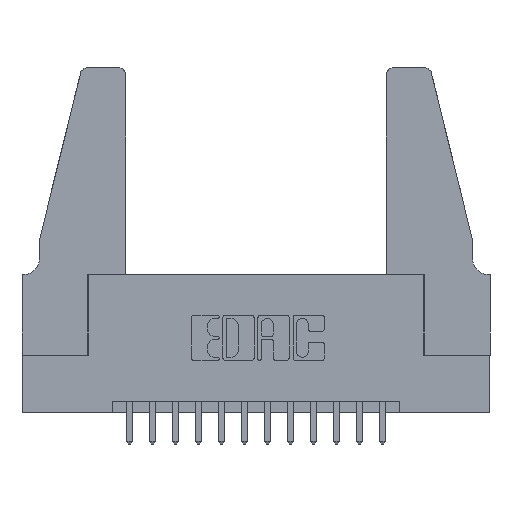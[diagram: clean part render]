
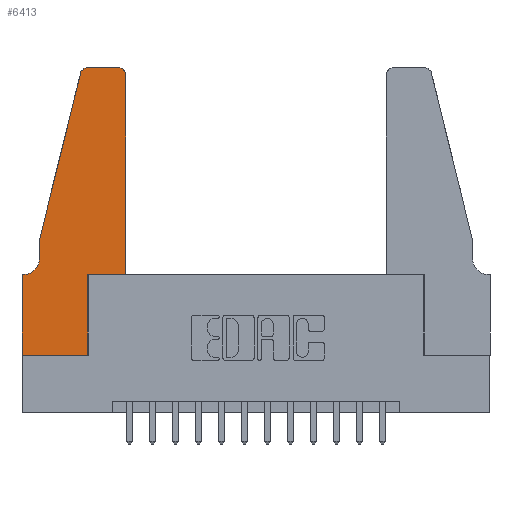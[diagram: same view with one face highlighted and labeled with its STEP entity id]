
A CAD part, top view. The second image highlights one B-rep face of the part: STEP entity #6413.
In plain terms, the highlighted planar face has unit normal (0, 0, 1).
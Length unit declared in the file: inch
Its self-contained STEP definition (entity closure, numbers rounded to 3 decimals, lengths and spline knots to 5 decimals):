
#133 = LINE ( 'NONE', #10324, #511 ) ;
#158 = EDGE_CURVE ( 'NONE', #15649, #6260, #133, .T. ) ;
#332 = EDGE_CURVE ( 'NONE', #9106, #620, #11481, .T. ) ;
#511 = VECTOR ( 'NONE', #10275, 39.37008 ) ;
#520 = VERTEX_POINT ( 'NONE', #4742 ) ;
#620 = VERTEX_POINT ( 'NONE', #6153 ) ;
#818 = EDGE_CURVE ( 'NONE', #14426, #7347, #7082, .T. ) ;
#876 = VECTOR ( 'NONE', #5156, 39.37008 ) ;
#976 = CARTESIAN_POINT ( 'NONE',  ( 0., 0.35, 0.37 ) ) ;
#988 = CARTESIAN_POINT ( 'NONE',  ( 0.4505, 0.35, 0.37 ) ) ;
#1846 = DIRECTION ( 'NONE',  ( 1., 0., 0. ) ) ;
#1961 = VECTOR ( 'NONE', #1846, 39.37008 ) ;
#2211 = CARTESIAN_POINT ( 'NONE',  ( 0.0755, 0.5, 0.37 ) ) ;
#2287 = LINE ( 'NONE', #13761, #9300 ) ;
#2394 = CARTESIAN_POINT ( 'NONE',  ( 0.2865, 0.35, 0.37 ) ) ;
#2395 = EDGE_CURVE ( 'NONE', #4177, #14426, #10451, .T. ) ;
#2438 = AXIS2_PLACEMENT_3D ( 'NONE', #7428, #11045, #14771 ) ;
#2499 = DIRECTION ( 'NONE',  ( 0., 1., 0. ) ) ;
#2516 = LINE ( 'NONE', #988, #14995 ) ;
#2868 = DIRECTION ( 'NONE',  ( 0., 0., 1. ) ) ;
#3017 = DIRECTION ( 'NONE',  ( 1., 0., 0. ) ) ;
#3064 = CARTESIAN_POINT ( 'NONE',  ( 0., 0., 0.37 ) ) ;
#3285 = VERTEX_POINT ( 'NONE', #8616 ) ;
#3447 = CARTESIAN_POINT ( 'NONE',  ( 0.4205, 1.25, 0.37 ) ) ;
#3520 = DIRECTION ( 'NONE',  ( -0.239, -0.971, 0. ) ) ;
#4177 = VERTEX_POINT ( 'NONE', #10153 ) ;
#4450 = CARTESIAN_POINT ( 'NONE',  ( 0.2865, 0.35, 0.37 ) ) ;
#4536 = PLANE ( 'NONE',  #8067 ) ;
#4601 = LINE ( 'NONE', #12689, #12036 ) ;
#4742 = CARTESIAN_POINT ( 'NONE',  ( 0.4505, 1.22, 0.37 ) ) ;
#4906 = DIRECTION ( 'NONE',  ( 1., 0., 0. ) ) ;
#4981 = VERTEX_POINT ( 'NONE', #6750 ) ;
#5156 = DIRECTION ( 'NONE',  ( 0., -1., 0. ) ) ;
#5166 = LINE ( 'NONE', #3064, #1961 ) ;
#5311 = CIRCLE ( 'NONE', #2438, 0.07 ) ;
#5348 = AXIS2_PLACEMENT_3D ( 'NONE', #7885, #2868, #3017 ) ;
#5444 = AXIS2_PLACEMENT_3D ( 'NONE', #10640, #8264, #9474 ) ;
#5755 = VERTEX_POINT ( 'NONE', #7774 ) ;
#5833 = ORIENTED_EDGE ( 'NONE', *, *, #13699, .T. ) ;
#6004 = ORIENTED_EDGE ( 'NONE', *, *, #12514, .T. ) ;
#6153 = CARTESIAN_POINT ( 'NONE',  ( 0.25487, 1.22718, 0.37 ) ) ;
#6260 = VERTEX_POINT ( 'NONE', #8727 ) ;
#6341 = ORIENTED_EDGE ( 'NONE', *, *, #818, .T. ) ;
#6383 = VERTEX_POINT ( 'NONE', #3447 ) ;
#6413 = ADVANCED_FACE ( 'NONE', ( #11841 ), #4536, .T. ) ;
#6750 = CARTESIAN_POINT ( 'NONE',  ( 0.0755, 0.42, 0.37 ) ) ;
#7082 = LINE ( 'NONE', #13169, #14453 ) ;
#7224 = VECTOR ( 'NONE', #2499, 39.37008 ) ;
#7321 = ORIENTED_EDGE ( 'NONE', *, *, #13750, .T. ) ;
#7347 = VERTEX_POINT ( 'NONE', #9357 ) ;
#7428 = CARTESIAN_POINT ( 'NONE',  ( 0.0055, 0.42, 0.37 ) ) ;
#7437 = EDGE_CURVE ( 'NONE', #7347, #520, #2516, .T. ) ;
#7774 = CARTESIAN_POINT ( 'NONE',  ( 0.0755, 0.5, 0.37 ) ) ;
#7885 = CARTESIAN_POINT ( 'NONE',  ( 0.4205, 1.22, 0.37 ) ) ;
#7935 = ORIENTED_EDGE ( 'NONE', *, *, #15416, .T. ) ;
#7985 = LINE ( 'NONE', #2211, #10629 ) ;
#8067 = AXIS2_PLACEMENT_3D ( 'NONE', #976, #9707, #4906 ) ;
#8264 = DIRECTION ( 'NONE',  ( 0., 0., 1. ) ) ;
#8502 = EDGE_CURVE ( 'NONE', #620, #5755, #7985, .T. ) ;
#8616 = CARTESIAN_POINT ( 'NONE',  ( 0., 0., 0.37 ) ) ;
#8701 = CARTESIAN_POINT ( 'NONE',  ( 0.0055, 0.35, 0.37 ) ) ;
#8727 = CARTESIAN_POINT ( 'NONE',  ( 0., 0.35, 0.37 ) ) ;
#9106 = VERTEX_POINT ( 'NONE', #11979 ) ;
#9300 = VECTOR ( 'NONE', #14984, 39.37008 ) ;
#9357 = CARTESIAN_POINT ( 'NONE',  ( 0.4505, 0.35, 0.37 ) ) ;
#9474 = DIRECTION ( 'NONE',  ( 1., 0., 0. ) ) ;
#9536 = ORIENTED_EDGE ( 'NONE', *, *, #8502, .T. ) ;
#9707 = DIRECTION ( 'NONE',  ( 0., 0., 1. ) ) ;
#10153 = CARTESIAN_POINT ( 'NONE',  ( 0.2865, 0., 0.37 ) ) ;
#10219 = ORIENTED_EDGE ( 'NONE', *, *, #15562, .T. ) ;
#10275 = DIRECTION ( 'NONE',  ( -1., 0., 0. ) ) ;
#10324 = CARTESIAN_POINT ( 'NONE',  ( 0.0755, 0.35, 0.37 ) ) ;
#10451 = LINE ( 'NONE', #2394, #7224 ) ;
#10583 = DIRECTION ( 'NONE',  ( 1., 0., 0. ) ) ;
#10629 = VECTOR ( 'NONE', #3520, 39.37008 ) ;
#10640 = CARTESIAN_POINT ( 'NONE',  ( 0.284, 1.22, 0.37 ) ) ;
#10669 = ORIENTED_EDGE ( 'NONE', *, *, #11886, .T. ) ;
#11045 = DIRECTION ( 'NONE',  ( 0., 0., -1. ) ) ;
#11481 = CIRCLE ( 'NONE', #5444, 0.03 ) ;
#11841 = FACE_OUTER_BOUND ( 'NONE', #14629, .T. ) ;
#11867 = CARTESIAN_POINT ( 'NONE',  ( 0.0755, 0.5, 0.37 ) ) ;
#11886 = EDGE_CURVE ( 'NONE', #5755, #4981, #14483, .T. ) ;
#11956 = ORIENTED_EDGE ( 'NONE', *, *, #2395, .T. ) ;
#11979 = CARTESIAN_POINT ( 'NONE',  ( 0.284, 1.25, 0.37 ) ) ;
#12036 = VECTOR ( 'NONE', #14989, 39.37008 ) ;
#12081 = ORIENTED_EDGE ( 'NONE', *, *, #7437, .T. ) ;
#12514 = EDGE_CURVE ( 'NONE', #6260, #3285, #4601, .T. ) ;
#12520 = ORIENTED_EDGE ( 'NONE', *, *, #158, .T. ) ;
#12689 = CARTESIAN_POINT ( 'NONE',  ( 0., 0., 0.37 ) ) ;
#13169 = CARTESIAN_POINT ( 'NONE',  ( 0.4505, 0.35, 0.37 ) ) ;
#13699 = EDGE_CURVE ( 'NONE', #520, #6383, #15604, .T. ) ;
#13750 = EDGE_CURVE ( 'NONE', #3285, #4177, #5166, .T. ) ;
#13761 = CARTESIAN_POINT ( 'NONE',  ( 0.2605, 1.25, 0.37 ) ) ;
#13779 = ORIENTED_EDGE ( 'NONE', *, *, #332, .T. ) ;
#14331 = DIRECTION ( 'NONE',  ( 0., 1., 0. ) ) ;
#14426 = VERTEX_POINT ( 'NONE', #4450 ) ;
#14453 = VECTOR ( 'NONE', #10583, 39.37008 ) ;
#14483 = LINE ( 'NONE', #11867, #876 ) ;
#14629 = EDGE_LOOP ( 'NONE', ( #10219, #13779, #9536, #10669, #7935, #12520, #6004, #7321, #11956, #6341, #12081, #5833 ) ) ;
#14771 = DIRECTION ( 'NONE',  ( -1., 0., 0. ) ) ;
#14984 = DIRECTION ( 'NONE',  ( -1., 0., 0. ) ) ;
#14989 = DIRECTION ( 'NONE',  ( 0., -1., 0. ) ) ;
#14995 = VECTOR ( 'NONE', #14331, 39.37008 ) ;
#15416 = EDGE_CURVE ( 'NONE', #4981, #15649, #5311, .T. ) ;
#15562 = EDGE_CURVE ( 'NONE', #6383, #9106, #2287, .T. ) ;
#15604 = CIRCLE ( 'NONE', #5348, 0.03 ) ;
#15649 = VERTEX_POINT ( 'NONE', #8701 ) ;
